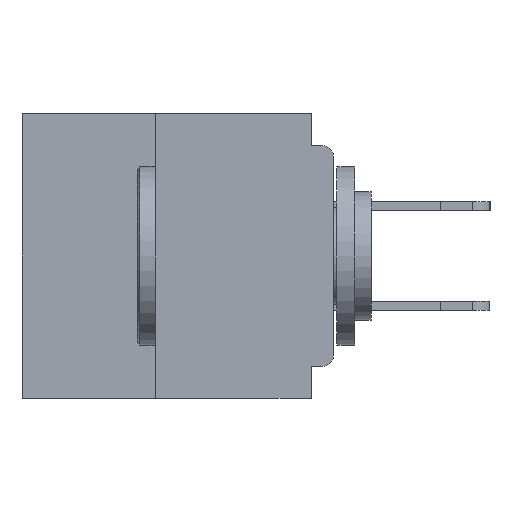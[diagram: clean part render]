
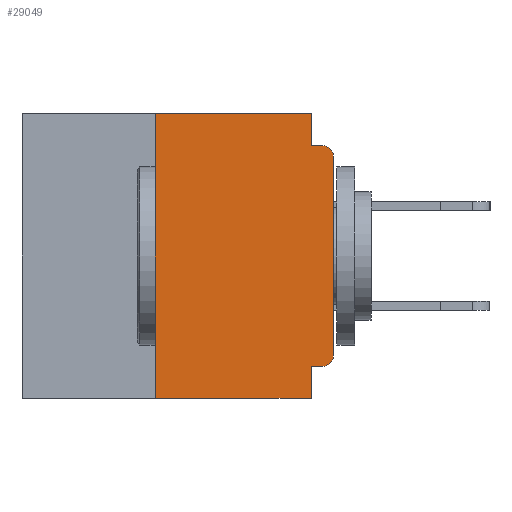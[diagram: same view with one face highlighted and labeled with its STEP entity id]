
A CAD part, left-side view. The second image highlights one B-rep face of the part: STEP entity #29049.
In plain terms, the highlighted planar face has unit normal (-1, 0, 0).
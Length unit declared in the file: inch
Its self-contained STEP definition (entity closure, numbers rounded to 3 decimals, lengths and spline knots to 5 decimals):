
#99 = ORIENTED_EDGE ( 'NONE', *, *, #31445, .T. ) ;
#752 = DIRECTION ( 'NONE',  ( 0., 0., -1. ) ) ;
#1153 = LINE ( 'NONE', #22824, #2220 ) ;
#1971 = VECTOR ( 'NONE', #33034, 39.37008 ) ;
#2220 = VECTOR ( 'NONE', #12767, 39.37008 ) ;
#2265 = CARTESIAN_POINT ( 'NONE',  ( 0., 0.25, -0.4 ) ) ;
#3482 = LINE ( 'NONE', #14345, #29026 ) ;
#3691 = VERTEX_POINT ( 'NONE', #21261 ) ;
#4145 = CARTESIAN_POINT ( 'NONE',  ( 0., 0.437, 0. ) ) ;
#4253 = ORIENTED_EDGE ( 'NONE', *, *, #22542, .F. ) ;
#6289 = VERTEX_POINT ( 'NONE', #8535 ) ;
#7402 = LINE ( 'NONE', #4145, #41823 ) ;
#8535 = CARTESIAN_POINT ( 'NONE',  ( 0., 0.015, -0.045 ) ) ;
#8791 = ORIENTED_EDGE ( 'NONE', *, *, #16626, .F. ) ;
#10506 = VERTEX_POINT ( 'NONE', #22522 ) ;
#10716 = ORIENTED_EDGE ( 'NONE', *, *, #39222, .T. ) ;
#10910 = CARTESIAN_POINT ( 'NONE',  ( 0., 0.437, 0. ) ) ;
#12125 = AXIS2_PLACEMENT_3D ( 'NONE', #34268, #14360, #37630 ) ;
#12284 = CIRCLE ( 'NONE', #35135, 0.015 ) ;
#12445 = LINE ( 'NONE', #13741, #21315 ) ;
#12728 = EDGE_CURVE ( 'NONE', #23055, #42840, #7402, .T. ) ;
#12767 = DIRECTION ( 'NONE',  ( 0., 0., 1. ) ) ;
#13108 = CARTESIAN_POINT ( 'NONE',  ( 0., 0.25, -0.4 ) ) ;
#13467 = CARTESIAN_POINT ( 'NONE',  ( 0., 0.25, 0. ) ) ;
#13741 = CARTESIAN_POINT ( 'NONE',  ( 0., 0.031, 0. ) ) ;
#13964 = CARTESIAN_POINT ( 'NONE',  ( 0., 0.031, -0.355 ) ) ;
#14304 = DIRECTION ( 'NONE',  ( 0., 0., -1. ) ) ;
#14345 = CARTESIAN_POINT ( 'NONE',  ( 0., 0., -0.045 ) ) ;
#14360 = DIRECTION ( 'NONE',  ( -1., 0., 0. ) ) ;
#15442 = FACE_OUTER_BOUND ( 'NONE', #18880, .T. ) ;
#15624 = DIRECTION ( 'NONE',  ( -1., 0., 0. ) ) ;
#15765 = CARTESIAN_POINT ( 'NONE',  ( 0., 0.015, -0.355 ) ) ;
#15947 = VECTOR ( 'NONE', #34726, 39.37008 ) ;
#16397 = LINE ( 'NONE', #37524, #16843 ) ;
#16626 = EDGE_CURVE ( 'NONE', #32432, #35528, #34689, .T. ) ;
#16831 = CIRCLE ( 'NONE', #12125, 0.015 ) ;
#16843 = VECTOR ( 'NONE', #752, 39.37008 ) ;
#17568 = DIRECTION ( 'NONE',  ( 0., -1., 0. ) ) ;
#18707 = LINE ( 'NONE', #13108, #1971 ) ;
#18880 = EDGE_LOOP ( 'NONE', ( #37699, #10716, #39639, #24324, #33064, #33910, #99, #4253, #8791, #38082 ) ) ;
#20415 = DIRECTION ( 'NONE',  ( 0., 0., -1. ) ) ;
#21029 = DIRECTION ( 'NONE',  ( 0., -1., 0. ) ) ;
#21261 = CARTESIAN_POINT ( 'NONE',  ( 0., 0., -0.34 ) ) ;
#21315 = VECTOR ( 'NONE', #20415, 39.37008 ) ;
#22137 = VECTOR ( 'NONE', #26594, 39.37008 ) ;
#22522 = CARTESIAN_POINT ( 'NONE',  ( 0., 0., -0.06 ) ) ;
#22542 = EDGE_CURVE ( 'NONE', #35528, #29461, #16397, .T. ) ;
#22824 = CARTESIAN_POINT ( 'NONE',  ( 0., 0., 0. ) ) ;
#23055 = VERTEX_POINT ( 'NONE', #13467 ) ;
#23068 = VERTEX_POINT ( 'NONE', #40289 ) ;
#24324 = ORIENTED_EDGE ( 'NONE', *, *, #26734, .F. ) ;
#25340 = EDGE_CURVE ( 'NONE', #35194, #23055, #18707, .T. ) ;
#26332 = CARTESIAN_POINT ( 'NONE',  ( 0., 0.031, -0.4 ) ) ;
#26594 = DIRECTION ( 'NONE',  ( 0., -1., 0. ) ) ;
#26734 = EDGE_CURVE ( 'NONE', #42840, #23068, #12445, .T. ) ;
#28180 = CARTESIAN_POINT ( 'NONE',  ( 0., 0., -0.355 ) ) ;
#29026 = VECTOR ( 'NONE', #21029, 39.37008 ) ;
#29049 = ADVANCED_FACE ( 'NONE', ( #15442 ), #30866, .F. ) ;
#29461 = VERTEX_POINT ( 'NONE', #26332 ) ;
#29945 = EDGE_CURVE ( 'NONE', #3691, #10506, #1153, .T. ) ;
#30866 = PLANE ( 'NONE',  #37535 ) ;
#31445 = EDGE_CURVE ( 'NONE', #35194, #29461, #32015, .T. ) ;
#32015 = LINE ( 'NONE', #39883, #22137 ) ;
#32432 = VERTEX_POINT ( 'NONE', #15765 ) ;
#33034 = DIRECTION ( 'NONE',  ( 0., 0., 1. ) ) ;
#33064 = ORIENTED_EDGE ( 'NONE', *, *, #12728, .F. ) ;
#33910 = ORIENTED_EDGE ( 'NONE', *, *, #25340, .F. ) ;
#34215 = DIRECTION ( 'NONE',  ( 1., 0., 0. ) ) ;
#34268 = CARTESIAN_POINT ( 'NONE',  ( 0., 0.015, -0.06 ) ) ;
#34689 = LINE ( 'NONE', #28180, #15947 ) ;
#34726 = DIRECTION ( 'NONE',  ( 0., 1., 0. ) ) ;
#35135 = AXIS2_PLACEMENT_3D ( 'NONE', #35551, #15624, #38922 ) ;
#35194 = VERTEX_POINT ( 'NONE', #2265 ) ;
#35528 = VERTEX_POINT ( 'NONE', #13964 ) ;
#35551 = CARTESIAN_POINT ( 'NONE',  ( 0., 0.015, -0.34 ) ) ;
#36247 = EDGE_CURVE ( 'NONE', #23068, #6289, #3482, .T. ) ;
#37524 = CARTESIAN_POINT ( 'NONE',  ( 0., 0.031, -0.4 ) ) ;
#37535 = AXIS2_PLACEMENT_3D ( 'NONE', #10910, #34215, #14304 ) ;
#37630 = DIRECTION ( 'NONE',  ( 0., 0., -1. ) ) ;
#37699 = ORIENTED_EDGE ( 'NONE', *, *, #29945, .T. ) ;
#38082 = ORIENTED_EDGE ( 'NONE', *, *, #42812, .T. ) ;
#38922 = DIRECTION ( 'NONE',  ( 0., 0., -1. ) ) ;
#39222 = EDGE_CURVE ( 'NONE', #10506, #6289, #16831, .T. ) ;
#39639 = ORIENTED_EDGE ( 'NONE', *, *, #36247, .F. ) ;
#39883 = CARTESIAN_POINT ( 'NONE',  ( 0., 0.437, -0.4 ) ) ;
#40289 = CARTESIAN_POINT ( 'NONE',  ( 0., 0.031, -0.045 ) ) ;
#41823 = VECTOR ( 'NONE', #17568, 39.37008 ) ;
#42299 = CARTESIAN_POINT ( 'NONE',  ( 0., 0.031, 0. ) ) ;
#42812 = EDGE_CURVE ( 'NONE', #32432, #3691, #12284, .T. ) ;
#42840 = VERTEX_POINT ( 'NONE', #42299 ) ;
